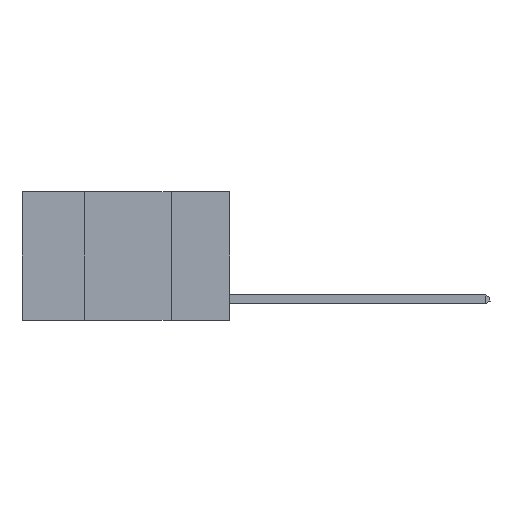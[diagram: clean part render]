
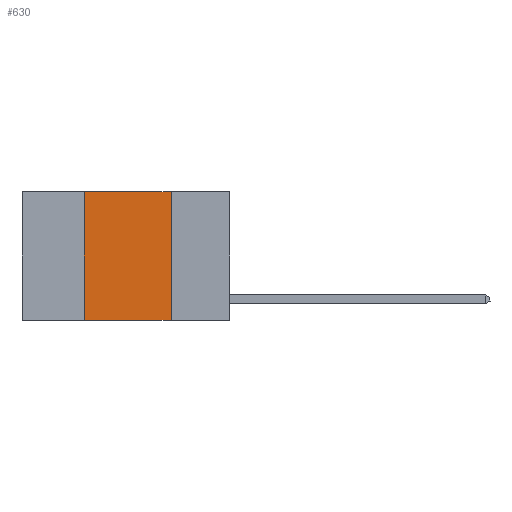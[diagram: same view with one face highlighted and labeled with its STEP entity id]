
A CAD part, left-side view. The second image highlights one B-rep face of the part: STEP entity #630.
In plain terms, the highlighted planar face has unit normal (-1, 0, 0).
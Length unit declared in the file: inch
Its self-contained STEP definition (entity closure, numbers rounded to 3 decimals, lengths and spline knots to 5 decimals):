
#219 = DIRECTION ( 'NONE',  ( 1., 0., 0. ) ) ;
#630 = ADVANCED_FACE ( 'NONE', ( #6251 ), #14422, .F. ) ;
#946 = VERTEX_POINT ( 'NONE', #7827 ) ;
#1550 = CARTESIAN_POINT ( 'NONE',  ( 0., 0.6, 0. ) ) ;
#2088 = EDGE_CURVE ( 'NONE', #16910, #946, #14090, .T. ) ;
#2520 = CARTESIAN_POINT ( 'NONE',  ( 0., 0.6, 0. ) ) ;
#2900 = CARTESIAN_POINT ( 'NONE',  ( 0., 0.17, 0. ) ) ;
#3739 = ORIENTED_EDGE ( 'NONE', *, *, #13552, .F. ) ;
#3918 = VECTOR ( 'NONE', #11285, 39.37008 ) ;
#4352 = LINE ( 'NONE', #2900, #17818 ) ;
#4563 = LINE ( 'NONE', #2520, #3918 ) ;
#4908 = EDGE_CURVE ( 'NONE', #11899, #946, #4352, .T. ) ;
#6251 = FACE_OUTER_BOUND ( 'NONE', #7706, .T. ) ;
#7706 = EDGE_LOOP ( 'NONE', ( #15011, #3739, #16453, #16265 ) ) ;
#7827 = CARTESIAN_POINT ( 'NONE',  ( 0., 0.17, -0.37 ) ) ;
#8714 = CARTESIAN_POINT ( 'NONE',  ( 0., 0.17, 0. ) ) ;
#8792 = DIRECTION ( 'NONE',  ( 0., 0., -1. ) ) ;
#9058 = VECTOR ( 'NONE', #16220, 39.37008 ) ;
#9166 = CARTESIAN_POINT ( 'NONE',  ( 0., 0.6, -0.37 ) ) ;
#10152 = CARTESIAN_POINT ( 'NONE',  ( 0., 0.42, -0.37 ) ) ;
#10168 = DIRECTION ( 'NONE',  ( 0., 0., -1. ) ) ;
#10171 = CARTESIAN_POINT ( 'NONE',  ( 0., 0.42, 0. ) ) ;
#10871 = EDGE_CURVE ( 'NONE', #16910, #15570, #16190, .T. ) ;
#11262 = AXIS2_PLACEMENT_3D ( 'NONE', #1550, #219, #10168 ) ;
#11285 = DIRECTION ( 'NONE',  ( 0., -1., 0. ) ) ;
#11899 = VERTEX_POINT ( 'NONE', #8714 ) ;
#13552 = EDGE_CURVE ( 'NONE', #15570, #11899, #4563, .T. ) ;
#14090 = LINE ( 'NONE', #9166, #9058 ) ;
#14422 = PLANE ( 'NONE',  #11262 ) ;
#14549 = DIRECTION ( 'NONE',  ( 0., 0., 1. ) ) ;
#15011 = ORIENTED_EDGE ( 'NONE', *, *, #4908, .F. ) ;
#15328 = VECTOR ( 'NONE', #14549, 39.37008 ) ;
#15570 = VERTEX_POINT ( 'NONE', #17347 ) ;
#16190 = LINE ( 'NONE', #10171, #15328 ) ;
#16220 = DIRECTION ( 'NONE',  ( 0., -1., 0. ) ) ;
#16265 = ORIENTED_EDGE ( 'NONE', *, *, #2088, .T. ) ;
#16453 = ORIENTED_EDGE ( 'NONE', *, *, #10871, .F. ) ;
#16910 = VERTEX_POINT ( 'NONE', #10152 ) ;
#17347 = CARTESIAN_POINT ( 'NONE',  ( 0., 0.42, 0. ) ) ;
#17818 = VECTOR ( 'NONE', #8792, 39.37008 ) ;
